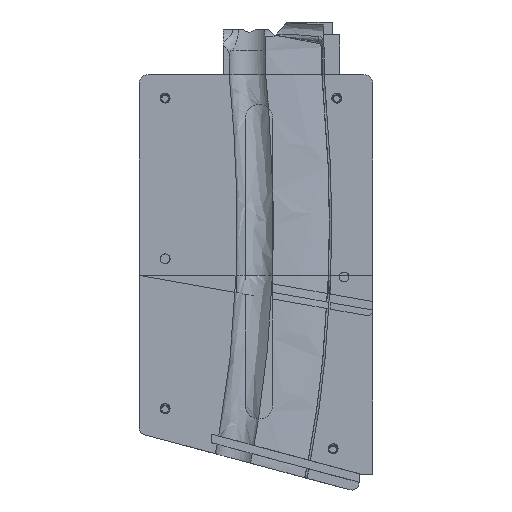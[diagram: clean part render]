
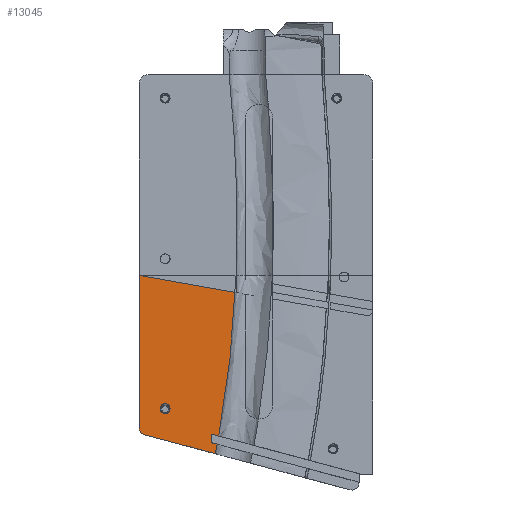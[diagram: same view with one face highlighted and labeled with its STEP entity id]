
A CAD part, front view. The second image highlights one B-rep face of the part: STEP entity #13045.
In plain terms, the highlighted planar face has unit normal (0, -1, 0).
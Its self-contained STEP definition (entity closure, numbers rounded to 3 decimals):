
#66=FACE_BOUND('',#1677,.T.);
#187=PLANE('',#13741);
#960=FACE_OUTER_BOUND('',#1676,.T.);
#1676=EDGE_LOOP('',(#11274,#11275,#11276,#11277,#11278,#11279,#11280,#11281,
#11282));
#1677=EDGE_LOOP('',(#11283,#11284,#11285,#11286));
#1890=CIRCLE('',#13669,1.5);
#1894=CIRCLE('',#13692,1.175);
#1902=CIRCLE('',#13742,2.);
#2836=B_SPLINE_CURVE_WITH_KNOTS('',3,(#137787,#137788,#137789,#137790),
 .UNSPECIFIED.,.F.,.F.,(4,4),(-9.92,-5.492),
 .UNSPECIFIED.);
#2841=B_SPLINE_CURVE_WITH_KNOTS('',3,(#138830,#138831,#138832,#138833,#138834,
#138835,#138836,#138837,#138838,#138839,#138840,#138841,#138842,#138843,
#138844,#138845),.UNSPECIFIED.,.F.,.F.,(4,2,2,2,2,2,2,4),(-0.436,
-0.383,-0.33,-0.251,-0.176,
-0.104,-0.047,0.),.UNSPECIFIED.);
#2856=B_SPLINE_CURVE_WITH_KNOTS('',3,(#140971,#140972,#140973,#140974,#140975,
#140976,#140977,#140978,#140979,#140980,#140981,#140982,#140983,#140984,
#140985,#140986),.UNSPECIFIED.,.F.,.F.,(4,2,2,2,2,2,2,4),(-0.243,
-0.225,-0.208,-0.174,-0.137,
-0.103,-0.058,0.),.UNSPECIFIED.);
#2881=B_SPLINE_CURVE_WITH_KNOTS('',3,(#142338,#142339,#142340,#142341),
 .UNSPECIFIED.,.F.,.F.,(4,4),(-10.412,-10.15),
 .UNSPECIFIED.);
#3678=LINE('',#137912,#4397);
#3679=LINE('',#138922,#4398);
#3686=LINE('',#138936,#4405);
#3693=LINE('',#142295,#4412);
#3701=LINE('',#142448,#4420);
#3708=LINE('',#142468,#4427);
#4397=VECTOR('',#15427,10.);
#4398=VECTOR('',#15432,10.);
#4405=VECTOR('',#15441,10.);
#4412=VECTOR('',#15472,10.);
#4420=VECTOR('',#15486,10.);
#4427=VECTOR('',#15505,10.);
#5527=VERTEX_POINT('',#134936);
#5528=VERTEX_POINT('',#134963);
#5571=VERTEX_POINT('',#136302);
#5572=VERTEX_POINT('',#136329);
#5618=VERTEX_POINT('',#137742);
#5619=VERTEX_POINT('',#137786);
#5623=VERTEX_POINT('',#137910);
#5625=VERTEX_POINT('',#138920);
#5626=VERTEX_POINT('',#138921);
#5632=VERTEX_POINT('',#138935);
#5659=VERTEX_POINT('',#142337);
#5662=VERTEX_POINT('',#142446);
#5666=VERTEX_POINT('',#142459);
#7376=EDGE_CURVE('',#5528,#5527,#1890,.T.);
#7436=EDGE_CURVE('',#5572,#5571,#1894,.T.);
#7502=EDGE_CURVE('',#5619,#5618,#2836,.T.);
#7508=EDGE_CURVE('',#5623,#5618,#3678,.T.);
#7511=EDGE_CURVE('',#5527,#5572,#2841,.T.);
#7515=EDGE_CURVE('',#5625,#5626,#3679,.F.);
#7522=EDGE_CURVE('',#5632,#5625,#3686,.T.);
#7540=EDGE_CURVE('',#5571,#5528,#2856,.T.);
#7567=EDGE_CURVE('',#5626,#5619,#3693,.F.);
#7573=EDGE_CURVE('',#5659,#5632,#2881,.T.);
#7579=EDGE_CURVE('',#5623,#5662,#3701,.T.);
#7589=EDGE_CURVE('',#5666,#5659,#3708,.T.);
#7590=EDGE_CURVE('',#5666,#5662,#1902,.T.);
#11274=ORIENTED_EDGE('',*,*,#7508,.F.);
#11275=ORIENTED_EDGE('',*,*,#7579,.T.);
#11276=ORIENTED_EDGE('',*,*,#7590,.F.);
#11277=ORIENTED_EDGE('',*,*,#7589,.T.);
#11278=ORIENTED_EDGE('',*,*,#7573,.T.);
#11279=ORIENTED_EDGE('',*,*,#7522,.T.);
#11280=ORIENTED_EDGE('',*,*,#7515,.T.);
#11281=ORIENTED_EDGE('',*,*,#7567,.T.);
#11282=ORIENTED_EDGE('',*,*,#7502,.T.);
#11283=ORIENTED_EDGE('',*,*,#7511,.T.);
#11284=ORIENTED_EDGE('',*,*,#7436,.T.);
#11285=ORIENTED_EDGE('',*,*,#7540,.T.);
#11286=ORIENTED_EDGE('',*,*,#7376,.T.);
#13045=ADVANCED_FACE('',(#960,#66),#187,.T.);
#13669=AXIS2_PLACEMENT_3D('',#134964,#15287,#15288);
#13692=AXIS2_PLACEMENT_3D('',#136330,#15352,#15353);
#13741=AXIS2_PLACEMENT_3D('',#142469,#15506,#15507);
#13742=AXIS2_PLACEMENT_3D('',#142470,#15508,#15509);
#15287=DIRECTION('center_axis',(0.,1.,0.));
#15288=DIRECTION('ref_axis',(1.,0.,0.));
#15352=DIRECTION('center_axis',(0.,1.,0.));
#15353=DIRECTION('ref_axis',(-1.,0.,0.));
#15427=DIRECTION('',(1.,0.,0.));
#15432=DIRECTION('',(0.,0.,-1.));
#15441=DIRECTION('',(-0.966,0.,0.259));
#15472=DIRECTION('',(-0.966,0.,0.259));
#15486=DIRECTION('',(0.,0.,-1.));
#15505=DIRECTION('',(0.966,0.,-0.259));
#15506=DIRECTION('center_axis',(0.,-1.,0.));
#15507=DIRECTION('ref_axis',(0.,0.,-1.));
#15508=DIRECTION('center_axis',(0.,1.,0.));
#15509=DIRECTION('ref_axis',(-0.793,0.,-0.609));
#134936=CARTESIAN_POINT('',(343.731,-27.877,-56.715));
#134963=CARTESIAN_POINT('',(342.571,-27.877,-56.792));
#134964=CARTESIAN_POINT('Origin',(343.243,-27.877,-58.134));
#136302=CARTESIAN_POINT('',(342.86,-27.877,-59.245));
#136329=CARTESIAN_POINT('',(343.769,-27.877,-59.185));
#136330=CARTESIAN_POINT('Origin',(343.243,-27.877,-58.134));
#137742=CARTESIAN_POINT('',(362.648,-27.877,-21.513));
#137786=CARTESIAN_POINT('',(357.916,-27.877,-65.481));
#137787=CARTESIAN_POINT('Ctrl Pts',(357.916,-27.877,
-65.481));
#137788=CARTESIAN_POINT('Ctrl Pts',(360.509,-27.877,
-51.211));
#137789=CARTESIAN_POINT('Ctrl Pts',(362.065,-27.877,
-36.638));
#137790=CARTESIAN_POINT('Ctrl Pts',(362.648,-27.877,
-21.513));
#137910=CARTESIAN_POINT('',(336.124,-27.877,-21.513));
#137912=CARTESIAN_POINT('',(368.119,-27.877,-21.513));
#138830=CARTESIAN_POINT('Ctrl Pts',(343.731,-27.877,-56.715));
#138831=CARTESIAN_POINT('Ctrl Pts',(343.831,-27.877,-56.761));
#138832=CARTESIAN_POINT('Ctrl Pts',(343.925,-27.877,
-56.817));
#138833=CARTESIAN_POINT('Ctrl Pts',(344.098,-27.877,
-56.948));
#138834=CARTESIAN_POINT('Ctrl Pts',(344.177,-27.877,-57.023));
#138835=CARTESIAN_POINT('Ctrl Pts',(344.35,-27.877,
-57.229));
#138836=CARTESIAN_POINT('Ctrl Pts',(344.444,-27.877,
-57.381));
#138837=CARTESIAN_POINT('Ctrl Pts',(344.562,-27.877,
-57.72));
#138838=CARTESIAN_POINT('Ctrl Pts',(344.587,-27.877,
-57.895));
#138839=CARTESIAN_POINT('Ctrl Pts',(344.566,-27.877,
-58.238));
#138840=CARTESIAN_POINT('Ctrl Pts',(344.524,-27.877,
-58.403));
#138841=CARTESIAN_POINT('Ctrl Pts',(344.395,-27.877,
-58.675));
#138842=CARTESIAN_POINT('Ctrl Pts',(344.306,-27.877,
-58.819));
#138843=CARTESIAN_POINT('Ctrl Pts',(344.05,-27.877,
-59.052));
#138844=CARTESIAN_POINT('Ctrl Pts',(343.915,-27.877,
-59.132));
#138845=CARTESIAN_POINT('Ctrl Pts',(343.769,-27.877,
-59.185));
#138920=CARTESIAN_POINT('',(355.887,-27.877,-67.318));
#138921=CARTESIAN_POINT('',(355.887,-27.877,-64.937));
#138922=CARTESIAN_POINT('',(355.887,-27.877,-40.686));
#138935=CARTESIAN_POINT('',(357.495,-27.877,-67.749));
#138936=CARTESIAN_POINT('',(366.245,-27.877,-70.093));
#140971=CARTESIAN_POINT('Ctrl Pts',(342.86,-27.877,
-59.245));
#140972=CARTESIAN_POINT('Ctrl Pts',(342.778,-27.877,
-59.227));
#140973=CARTESIAN_POINT('Ctrl Pts',(342.698,-27.877,
-59.201));
#140974=CARTESIAN_POINT('Ctrl Pts',(342.543,-27.877,
-59.131));
#140975=CARTESIAN_POINT('Ctrl Pts',(342.469,-27.877,
-59.088));
#140976=CARTESIAN_POINT('Ctrl Pts',(342.267,-27.877,
-58.938));
#140977=CARTESIAN_POINT('Ctrl Pts',(342.16,-27.877,
-58.816));
#140978=CARTESIAN_POINT('Ctrl Pts',(341.986,-27.877,
-58.523));
#140979=CARTESIAN_POINT('Ctrl Pts',(341.926,-27.877,
-58.355));
#140980=CARTESIAN_POINT('Ctrl Pts',(341.878,-27.877,
-58.017));
#140981=CARTESIAN_POINT('Ctrl Pts',(341.885,-27.877,
-57.85));
#140982=CARTESIAN_POINT('Ctrl Pts',(341.972,-27.877,
-57.476));
#140983=CARTESIAN_POINT('Ctrl Pts',(342.066,-27.877,
-57.306));
#140984=CARTESIAN_POINT('Ctrl Pts',(342.267,-27.877,
-57.027));
#140985=CARTESIAN_POINT('Ctrl Pts',(342.408,-27.877,
-56.894));
#140986=CARTESIAN_POINT('Ctrl Pts',(342.571,-27.877,
-56.792));
#142295=CARTESIAN_POINT('',(366.84,-27.877,-67.872));
#142337=CARTESIAN_POINT('',(356.991,-27.877,-70.337));
#142338=CARTESIAN_POINT('Ctrl Pts',(356.991,-27.877,
-70.337));
#142339=CARTESIAN_POINT('Ctrl Pts',(357.163,-27.877,
-69.475));
#142340=CARTESIAN_POINT('Ctrl Pts',(357.331,-27.877,
-68.613));
#142341=CARTESIAN_POINT('Ctrl Pts',(357.495,-27.877,
-67.749));
#142446=CARTESIAN_POINT('',(336.124,-27.877,-63.211));
#142448=CARTESIAN_POINT('',(336.124,-27.877,-38.016));
#142459=CARTESIAN_POINT('',(337.606,-27.877,-65.143));
#142468=CARTESIAN_POINT('',(353.859,-27.877,-69.498));
#142469=CARTESIAN_POINT('Origin',(368.119,-27.877,-15.178));
#142470=CARTESIAN_POINT('Origin',(338.124,-27.877,-63.211));
